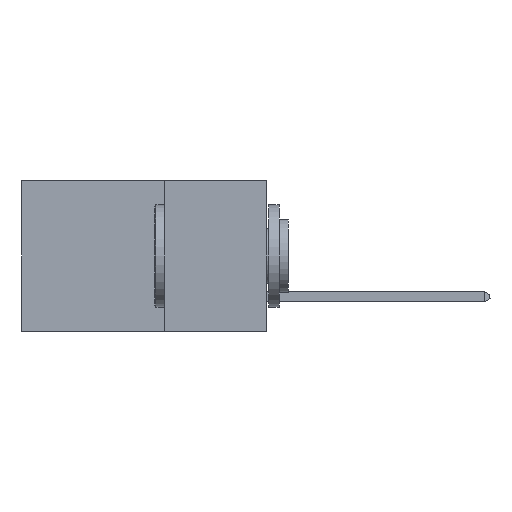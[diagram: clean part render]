
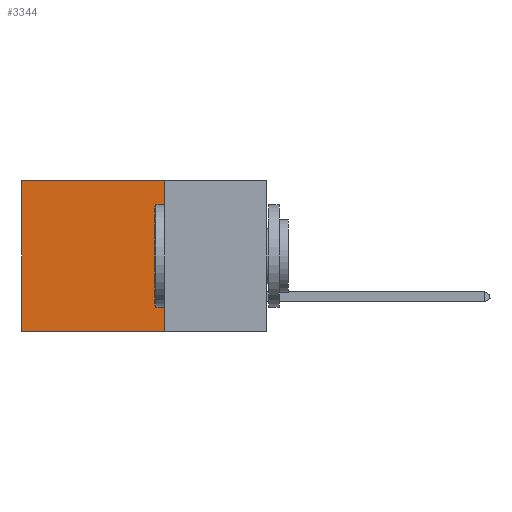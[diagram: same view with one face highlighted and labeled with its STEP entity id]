
A CAD part, left-side view. The second image highlights one B-rep face of the part: STEP entity #3344.
In plain terms, the highlighted planar face has unit normal (-1, 0, 0).
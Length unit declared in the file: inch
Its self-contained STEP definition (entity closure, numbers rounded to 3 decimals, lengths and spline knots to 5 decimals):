
#518 = FACE_OUTER_BOUND ( 'NONE', #1107, .T. ) ;
#736 = LINE ( 'NONE', #8560, #8004 ) ;
#1040 = LINE ( 'NONE', #15875, #14543 ) ;
#1107 = EDGE_LOOP ( 'NONE', ( #2230, #8171, #16682, #9066 ) ) ;
#1144 = VERTEX_POINT ( 'NONE', #15853 ) ;
#2230 = ORIENTED_EDGE ( 'NONE', *, *, #17519, .T. ) ;
#3126 = CARTESIAN_POINT ( 'NONE',  ( 0.2875, 0.25, 0. ) ) ;
#3344 = ADVANCED_FACE ( 'NONE', ( #518 ), #3453, .F. ) ;
#3453 = PLANE ( 'NONE',  #18307 ) ;
#3572 = EDGE_CURVE ( 'NONE', #4293, #1144, #17303, .T. ) ;
#4123 = VERTEX_POINT ( 'NONE', #9421 ) ;
#4293 = VERTEX_POINT ( 'NONE', #12319 ) ;
#4333 = VECTOR ( 'NONE', #11605, 39.37008 ) ;
#5740 = LINE ( 'NONE', #10193, #4333 ) ;
#5979 = DIRECTION ( 'NONE',  ( 0., 1., 0. ) ) ;
#7629 = EDGE_CURVE ( 'NONE', #4293, #17617, #5740, .T. ) ;
#8004 = VECTOR ( 'NONE', #8758, 39.37008 ) ;
#8171 = ORIENTED_EDGE ( 'NONE', *, *, #8304, .F. ) ;
#8304 = EDGE_CURVE ( 'NONE', #17617, #4123, #736, .T. ) ;
#8560 = CARTESIAN_POINT ( 'NONE',  ( 0.2875, 0.25, -0.37 ) ) ;
#8758 = DIRECTION ( 'NONE',  ( 0., 1., 0. ) ) ;
#9066 = ORIENTED_EDGE ( 'NONE', *, *, #3572, .T. ) ;
#9421 = CARTESIAN_POINT ( 'NONE',  ( 0.2875, 0.6, -0.37 ) ) ;
#9565 = DIRECTION ( 'NONE',  ( 0., 0., -1. ) ) ;
#10193 = CARTESIAN_POINT ( 'NONE',  ( 0.2875, 0.25, 0. ) ) ;
#11605 = DIRECTION ( 'NONE',  ( 0., 0., -1. ) ) ;
#12285 = CARTESIAN_POINT ( 'NONE',  ( 0.2875, 0.25, 0. ) ) ;
#12319 = CARTESIAN_POINT ( 'NONE',  ( 0.2875, 0.25, 0. ) ) ;
#12632 = VECTOR ( 'NONE', #5979, 39.37008 ) ;
#14543 = VECTOR ( 'NONE', #17312, 39.37008 ) ;
#14627 = CARTESIAN_POINT ( 'NONE',  ( 0.2875, 0.25, -0.37 ) ) ;
#15467 = DIRECTION ( 'NONE',  ( 1., 0., 0. ) ) ;
#15853 = CARTESIAN_POINT ( 'NONE',  ( 0.2875, 0.6, 0. ) ) ;
#15875 = CARTESIAN_POINT ( 'NONE',  ( 0.2875, 0.6, 0. ) ) ;
#16682 = ORIENTED_EDGE ( 'NONE', *, *, #7629, .F. ) ;
#17303 = LINE ( 'NONE', #3126, #12632 ) ;
#17312 = DIRECTION ( 'NONE',  ( 0., 0., -1. ) ) ;
#17519 = EDGE_CURVE ( 'NONE', #1144, #4123, #1040, .T. ) ;
#17617 = VERTEX_POINT ( 'NONE', #14627 ) ;
#18307 = AXIS2_PLACEMENT_3D ( 'NONE', #12285, #15467, #9565 ) ;
